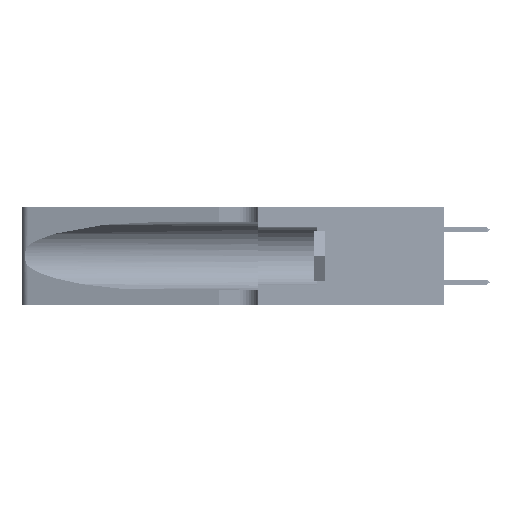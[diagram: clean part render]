
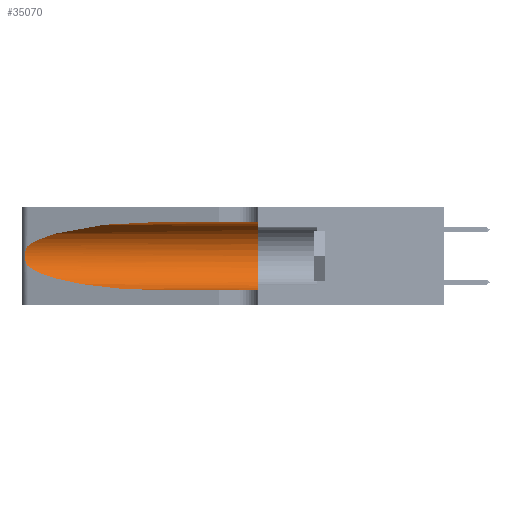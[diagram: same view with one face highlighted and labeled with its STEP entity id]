
A CAD part, left-side view. The second image highlights one B-rep face of the part: STEP entity #35070.
In plain terms, the highlighted cylindrical face has radius 3.308 mm (diameter 6.617 mm), a partial arc.
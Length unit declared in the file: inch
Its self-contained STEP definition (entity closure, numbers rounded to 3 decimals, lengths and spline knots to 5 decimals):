
#1556 = CARTESIAN_POINT ( 'NONE',  ( 0.1305, 1.61858, 0.31525 ) ) ;
#1978 = CARTESIAN_POINT ( 'NONE',  ( 0.25787, 1.23484, 0.2124 ) ) ;
#2708 = ORIENTED_EDGE ( 'NONE', *, *, #34393, .T. ) ;
#2855 = ORIENTED_EDGE ( 'NONE', *, *, #43351, .F. ) ;
#2937 = DIRECTION ( 'NONE',  ( 0., 0., -1. ) ) ;
#3292 = LINE ( 'NONE', #1556, #22901 ) ;
#4024 = B_SPLINE_CURVE_WITH_KNOTS ( 'NONE', 3,
 ( #42410, #16663, #24065, #1978, #27754, #5680, #31454, #9400, #35153, #13136, #38862, #16812, #42576, #20515 ),
 .UNSPECIFIED., .F., .F.,
 ( 4, 2, 2, 2, 2, 2, 4 ),
 ( 0., 0.00027, 0.00053, 0.00107, 0.0016, 0.00187, 0.00214 ),
 .UNSPECIFIED. ) ;
#5680 = CARTESIAN_POINT ( 'NONE',  ( 0.26018, 1.23835, 0.19895 ) ) ;
#5886 = DIRECTION ( 'NONE',  ( 0., 1., 0. ) ) ;
#8804 = CARTESIAN_POINT ( 'NONE',  ( 0.1305, 0.72297, 0.05475 ) ) ;
#9400 = CARTESIAN_POINT ( 'NONE',  ( 0.26075, 1.23896, 0.178 ) ) ;
#12644 =( BOUNDED_CURVE ( )  B_SPLINE_CURVE ( 3, ( #43437, #35999, #14150, #39873 ),
 .UNSPECIFIED., .F., .F. ) 
 B_SPLINE_CURVE_WITH_KNOTS ( ( 4, 4 ),
 ( 1.5708, 2.84003 ),
 .UNSPECIFIED. ) 
 CURVE ( )  GEOMETRIC_REPRESENTATION_ITEM ( )  RATIONAL_B_SPLINE_CURVE ( ( 1., 0.87, 0.87, 1. ) ) 
 REPRESENTATION_ITEM ( '' )  );
#12835 = CIRCLE ( 'NONE', #17274, 0.13025 ) ;
#13136 = CARTESIAN_POINT ( 'NONE',  ( 0.25856, 1.23593, 0.16098 ) ) ;
#13946 = DIRECTION ( 'NONE',  ( 0., -1., 0. ) ) ;
#13988 = VERTEX_POINT ( 'NONE', #25389 ) ;
#14150 = CARTESIAN_POINT ( 'NONE',  ( 0.2373, 1.15595, 0.28018 ) ) ;
#14866 = DIRECTION ( 'NONE',  ( 0., -1., 0. ) ) ;
#16058 = CARTESIAN_POINT ( 'NONE',  ( 0.2373, 1.15595, 0.08982 ) ) ;
#16140 = CARTESIAN_POINT ( 'NONE',  ( 0.1305, 0.72297, 0.31525 ) ) ;
#16663 = CARTESIAN_POINT ( 'NONE',  ( 0.25555, 1.22994, 0.2215 ) ) ;
#16687 = LINE ( 'NONE', #22270, #36245 ) ;
#16812 = CARTESIAN_POINT ( 'NONE',  ( 0.25639, 1.23186, 0.15144 ) ) ;
#17274 = AXIS2_PLACEMENT_3D ( 'NONE', #27962, #5886, #31662 ) ;
#18449 = CARTESIAN_POINT ( 'NONE',  ( 0.1305, 0.35, 0.31525 ) ) ;
#20261 = EDGE_CURVE ( 'NONE', #31332, #46287, #12835, .T. ) ;
#20515 = CARTESIAN_POINT ( 'NONE',  ( 0.25487, 1.22718, 0.14631 ) ) ;
#21751 = EDGE_CURVE ( 'NONE', #35887, #46287, #16687, .T. ) ;
#21859 = EDGE_LOOP ( 'NONE', ( #2708, #21862, #23581, #41067, #29785, #2855 ) ) ;
#21862 = ORIENTED_EDGE ( 'NONE', *, *, #36542, .T. ) ;
#22270 = CARTESIAN_POINT ( 'NONE',  ( 0.1305, 1.61858, 0.05475 ) ) ;
#22901 = VECTOR ( 'NONE', #27326, 39.37008 ) ;
#23581 = ORIENTED_EDGE ( 'NONE', *, *, #40571, .T. ) ;
#23849 = AXIS2_PLACEMENT_3D ( 'NONE', #25033, #13946, #2937 ) ;
#23980 = VERTEX_POINT ( 'NONE', #16140 ) ;
#24065 = CARTESIAN_POINT ( 'NONE',  ( 0.25639, 1.23184, 0.21858 ) ) ;
#25033 = CARTESIAN_POINT ( 'NONE',  ( 0.1305, 1.61858, 0.185 ) ) ;
#25389 = CARTESIAN_POINT ( 'NONE',  ( 0.25487, 1.22718, 0.14631 ) ) ;
#27326 = DIRECTION ( 'NONE',  ( 0., -1., 0. ) ) ;
#27754 = CARTESIAN_POINT ( 'NONE',  ( 0.25854, 1.2359, 0.20912 ) ) ;
#27962 = CARTESIAN_POINT ( 'NONE',  ( 0.1305, 0.35, 0.185 ) ) ;
#28455 = FACE_OUTER_BOUND ( 'NONE', #21859, .T. ) ;
#28837 = VERTEX_POINT ( 'NONE', #46146 ) ;
#29785 = ORIENTED_EDGE ( 'NONE', *, *, #20261, .F. ) ;
#30094 = CARTESIAN_POINT ( 'NONE',  ( 0.1305, 0.72297, 0.05475 ) ) ;
#30871 = CARTESIAN_POINT ( 'NONE',  ( 0.18966, 0.96281, 0.05475 ) ) ;
#31332 = VERTEX_POINT ( 'NONE', #18449 ) ;
#31454 = CARTESIAN_POINT ( 'NONE',  ( 0.26075, 1.23896, 0.19203 ) ) ;
#31662 = DIRECTION ( 'NONE',  ( 0., 0., 1. ) ) ;
#34393 = EDGE_CURVE ( 'NONE', #23980, #28837, #12644, .T. ) ;
#34754 =( BOUNDED_CURVE ( )  B_SPLINE_CURVE ( 3, ( #45532, #16058, #30871, #8804 ),
 .UNSPECIFIED., .F., .F. ) 
 B_SPLINE_CURVE_WITH_KNOTS ( ( 4, 4 ),
 ( 3.44316, 4.71239 ),
 .UNSPECIFIED. ) 
 CURVE ( )  GEOMETRIC_REPRESENTATION_ITEM ( )  RATIONAL_B_SPLINE_CURVE ( ( 1., 0.87, 0.87, 1. ) ) 
 REPRESENTATION_ITEM ( '' )  );
#35070 = ADVANCED_FACE ( 'NONE', ( #28455 ), #37064, .F. ) ;
#35153 = CARTESIAN_POINT ( 'NONE',  ( 0.26017, 1.23833, 0.17102 ) ) ;
#35887 = VERTEX_POINT ( 'NONE', #30094 ) ;
#35999 = CARTESIAN_POINT ( 'NONE',  ( 0.18966, 0.96281, 0.31525 ) ) ;
#36245 = VECTOR ( 'NONE', #14866, 39.37008 ) ;
#36542 = EDGE_CURVE ( 'NONE', #28837, #13988, #4024, .T. ) ;
#37064 = CYLINDRICAL_SURFACE ( 'NONE', #23849, 0.13025 ) ;
#38862 = CARTESIAN_POINT ( 'NONE',  ( 0.25789, 1.23486, 0.15765 ) ) ;
#39873 = CARTESIAN_POINT ( 'NONE',  ( 0.25487, 1.22718, 0.22369 ) ) ;
#40571 = EDGE_CURVE ( 'NONE', #13988, #35887, #34754, .T. ) ;
#41067 = ORIENTED_EDGE ( 'NONE', *, *, #21751, .T. ) ;
#42410 = CARTESIAN_POINT ( 'NONE',  ( 0.25487, 1.22718, 0.22369 ) ) ;
#42576 = CARTESIAN_POINT ( 'NONE',  ( 0.25555, 1.22993, 0.14849 ) ) ;
#43351 = EDGE_CURVE ( 'NONE', #23980, #31332, #3292, .T. ) ;
#43437 = CARTESIAN_POINT ( 'NONE',  ( 0.1305, 0.72297, 0.31525 ) ) ;
#45417 = CARTESIAN_POINT ( 'NONE',  ( 0.1305, 0.35, 0.05475 ) ) ;
#45532 = CARTESIAN_POINT ( 'NONE',  ( 0.25487, 1.22718, 0.14631 ) ) ;
#46146 = CARTESIAN_POINT ( 'NONE',  ( 0.25487, 1.22718, 0.22369 ) ) ;
#46287 = VERTEX_POINT ( 'NONE', #45417 ) ;
